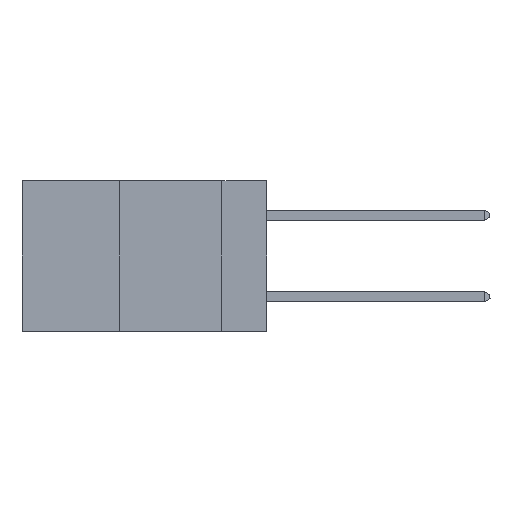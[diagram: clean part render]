
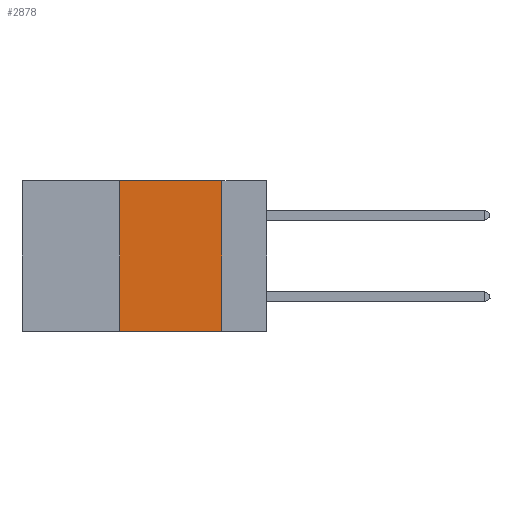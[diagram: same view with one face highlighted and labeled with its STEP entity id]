
A CAD part, left-side view. The second image highlights one B-rep face of the part: STEP entity #2878.
In plain terms, the highlighted planar face has unit normal (-1, 0, 0).
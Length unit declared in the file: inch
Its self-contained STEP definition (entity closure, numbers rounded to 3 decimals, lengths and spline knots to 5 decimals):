
#296 = VECTOR ( 'NONE', #12664, 39.37008 ) ;
#547 = CARTESIAN_POINT ( 'NONE',  ( 0., 0.6, 0. ) ) ;
#1838 = VERTEX_POINT ( 'NONE', #25570 ) ;
#1991 = CARTESIAN_POINT ( 'NONE',  ( 0., 0.36, 0. ) ) ;
#2878 = ADVANCED_FACE ( 'NONE', ( #6629 ), #10137, .F. ) ;
#3430 = EDGE_CURVE ( 'NONE', #16676, #25693, #29959, .T. ) ;
#4803 = EDGE_CURVE ( 'NONE', #1838, #25136, #20399, .T. ) ;
#5680 = CARTESIAN_POINT ( 'NONE',  ( 0., 0.11, 0. ) ) ;
#6572 = VECTOR ( 'NONE', #9272, 39.37008 ) ;
#6629 = FACE_OUTER_BOUND ( 'NONE', #14916, .T. ) ;
#9272 = DIRECTION ( 'NONE',  ( 0., 0., 1. ) ) ;
#10137 = PLANE ( 'NONE',  #17666 ) ;
#10715 = LINE ( 'NONE', #1991, #6572 ) ;
#12664 = DIRECTION ( 'NONE',  ( 0., 0., -1. ) ) ;
#14916 = EDGE_LOOP ( 'NONE', ( #23194, #30096, #15012, #30105 ) ) ;
#15012 = ORIENTED_EDGE ( 'NONE', *, *, #24280, .F. ) ;
#15468 = CARTESIAN_POINT ( 'NONE',  ( 0., 0.6, 0. ) ) ;
#15782 = CARTESIAN_POINT ( 'NONE',  ( 0., 0.6, -0.37 ) ) ;
#16676 = VERTEX_POINT ( 'NONE', #28794 ) ;
#17076 = DIRECTION ( 'NONE',  ( 0., 0., -1. ) ) ;
#17666 = AXIS2_PLACEMENT_3D ( 'NONE', #547, #21969, #17076 ) ;
#20399 = LINE ( 'NONE', #15468, #24927 ) ;
#20632 = LINE ( 'NONE', #5680, #296 ) ;
#21802 = CARTESIAN_POINT ( 'NONE',  ( 0., 0.11, -0.37 ) ) ;
#21969 = DIRECTION ( 'NONE',  ( 1., 0., 0. ) ) ;
#23194 = ORIENTED_EDGE ( 'NONE', *, *, #28779, .F. ) ;
#24280 = EDGE_CURVE ( 'NONE', #16676, #1838, #10715, .T. ) ;
#24611 = VECTOR ( 'NONE', #30184, 39.37008 ) ;
#24927 = VECTOR ( 'NONE', #30082, 39.37008 ) ;
#25136 = VERTEX_POINT ( 'NONE', #30984 ) ;
#25570 = CARTESIAN_POINT ( 'NONE',  ( 0., 0.36, 0. ) ) ;
#25693 = VERTEX_POINT ( 'NONE', #21802 ) ;
#28779 = EDGE_CURVE ( 'NONE', #25136, #25693, #20632, .T. ) ;
#28794 = CARTESIAN_POINT ( 'NONE',  ( 0., 0.36, -0.37 ) ) ;
#29959 = LINE ( 'NONE', #15782, #24611 ) ;
#30082 = DIRECTION ( 'NONE',  ( 0., -1., 0. ) ) ;
#30096 = ORIENTED_EDGE ( 'NONE', *, *, #4803, .F. ) ;
#30105 = ORIENTED_EDGE ( 'NONE', *, *, #3430, .T. ) ;
#30184 = DIRECTION ( 'NONE',  ( 0., -1., 0. ) ) ;
#30984 = CARTESIAN_POINT ( 'NONE',  ( 0., 0.11, 0. ) ) ;
